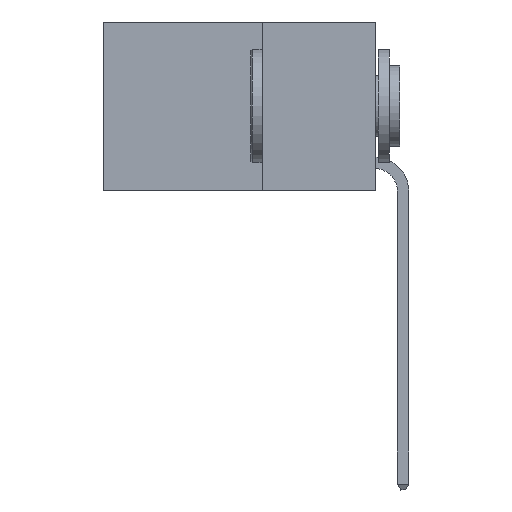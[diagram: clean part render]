
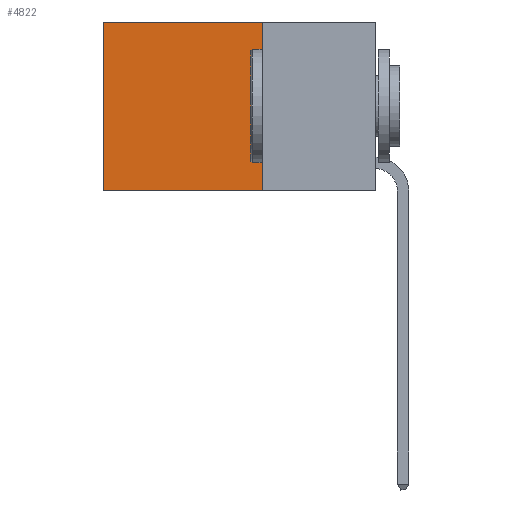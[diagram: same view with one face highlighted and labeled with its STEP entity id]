
A CAD part, left-side view. The second image highlights one B-rep face of the part: STEP entity #4822.
In plain terms, the highlighted planar face has unit normal (-1, 0, 0).
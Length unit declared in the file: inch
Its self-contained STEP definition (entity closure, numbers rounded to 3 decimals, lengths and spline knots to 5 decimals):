
#44 = LINE ( 'NONE', #4854, #26225 ) ;
#82 = CARTESIAN_POINT ( 'NONE',  ( 0.2625, 0.25, 0. ) ) ;
#1235 = DIRECTION ( 'NONE',  ( 1., 0., 0. ) ) ;
#1880 = CARTESIAN_POINT ( 'NONE',  ( 0.2625, 0.6, 0. ) ) ;
#2935 = CARTESIAN_POINT ( 'NONE',  ( 0.2625, 0.6, 0. ) ) ;
#2955 = VERTEX_POINT ( 'NONE', #7980 ) ;
#4822 = ADVANCED_FACE ( 'NONE', ( #8420 ), #29267, .F. ) ;
#4854 = CARTESIAN_POINT ( 'NONE',  ( 0.2625, 0.25, 0. ) ) ;
#7731 = CARTESIAN_POINT ( 'NONE',  ( 0.2625, 0.25, 0. ) ) ;
#7980 = CARTESIAN_POINT ( 'NONE',  ( 0.2625, 0.25, -0.37 ) ) ;
#8420 = FACE_OUTER_BOUND ( 'NONE', #22147, .T. ) ;
#9829 = LINE ( 'NONE', #7731, #23842 ) ;
#10528 = DIRECTION ( 'NONE',  ( 0., 0., -1. ) ) ;
#10630 = ORIENTED_EDGE ( 'NONE', *, *, #19117, .F. ) ;
#11899 = VECTOR ( 'NONE', #13007, 39.37008 ) ;
#13007 = DIRECTION ( 'NONE',  ( 0., 0., -1. ) ) ;
#13614 = DIRECTION ( 'NONE',  ( 0., 1., 0. ) ) ;
#14971 = EDGE_CURVE ( 'NONE', #19130, #20331, #44, .T. ) ;
#15557 = ORIENTED_EDGE ( 'NONE', *, *, #22689, .F. ) ;
#15605 = VECTOR ( 'NONE', #13614, 39.37008 ) ;
#18849 = CARTESIAN_POINT ( 'NONE',  ( 0.2625, 0.6, -0.37 ) ) ;
#19017 = DIRECTION ( 'NONE',  ( 0., 0., -1. ) ) ;
#19117 = EDGE_CURVE ( 'NONE', #2955, #27225, #23070, .T. ) ;
#19130 = VERTEX_POINT ( 'NONE', #82 ) ;
#20331 = VERTEX_POINT ( 'NONE', #2935 ) ;
#22147 = EDGE_LOOP ( 'NONE', ( #24656, #10630, #15557, #28472 ) ) ;
#22159 = LINE ( 'NONE', #1880, #11899 ) ;
#22396 = CARTESIAN_POINT ( 'NONE',  ( 0.2625, 0.25, 0. ) ) ;
#22689 = EDGE_CURVE ( 'NONE', #19130, #2955, #9829, .T. ) ;
#23070 = LINE ( 'NONE', #27851, #15605 ) ;
#23842 = VECTOR ( 'NONE', #19017, 39.37008 ) ;
#24656 = ORIENTED_EDGE ( 'NONE', *, *, #25432, .T. ) ;
#24984 = DIRECTION ( 'NONE',  ( 0., 1., 0. ) ) ;
#25432 = EDGE_CURVE ( 'NONE', #20331, #27225, #22159, .T. ) ;
#26225 = VECTOR ( 'NONE', #24984, 39.37008 ) ;
#26409 = AXIS2_PLACEMENT_3D ( 'NONE', #22396, #1235, #10528 ) ;
#27225 = VERTEX_POINT ( 'NONE', #18849 ) ;
#27851 = CARTESIAN_POINT ( 'NONE',  ( 0.2625, 0.25, -0.37 ) ) ;
#28472 = ORIENTED_EDGE ( 'NONE', *, *, #14971, .T. ) ;
#29267 = PLANE ( 'NONE',  #26409 ) ;
